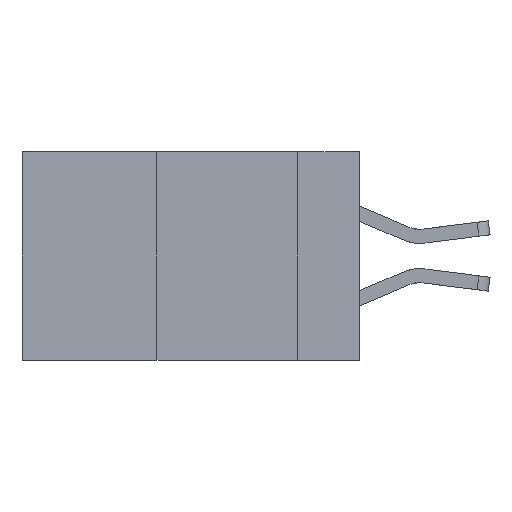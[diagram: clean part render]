
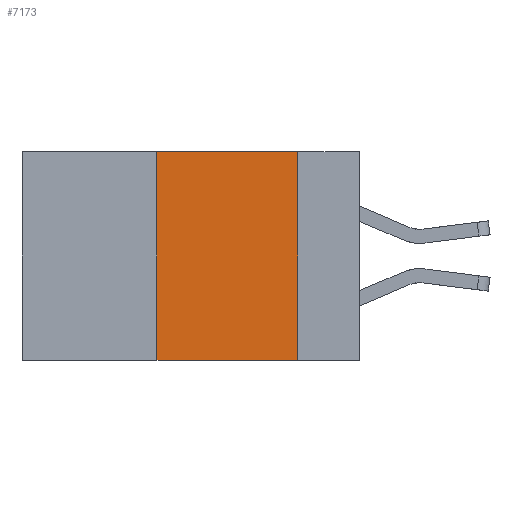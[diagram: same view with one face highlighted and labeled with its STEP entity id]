
A CAD part, left-side view. The second image highlights one B-rep face of the part: STEP entity #7173.
In plain terms, the highlighted planar face has unit normal (-1, 0, 0).
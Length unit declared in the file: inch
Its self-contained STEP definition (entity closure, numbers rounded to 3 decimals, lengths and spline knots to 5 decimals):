
#502 = DIRECTION ( 'NONE',  ( 0., -1., 0. ) ) ;
#1056 = DIRECTION ( 'NONE',  ( 0., -1., 0. ) ) ;
#1203 = CARTESIAN_POINT ( 'NONE',  ( 0., 0.11, 0. ) ) ;
#1405 = VECTOR ( 'NONE', #502, 39.37008 ) ;
#1530 = ORIENTED_EDGE ( 'NONE', *, *, #6728, .F. ) ;
#1878 = PLANE ( 'NONE',  #2097 ) ;
#2097 = AXIS2_PLACEMENT_3D ( 'NONE', #2658, #3518, #3548 ) ;
#2398 = ORIENTED_EDGE ( 'NONE', *, *, #4056, .T. ) ;
#2619 = ORIENTED_EDGE ( 'NONE', *, *, #3379, .F. ) ;
#2658 = CARTESIAN_POINT ( 'NONE',  ( 0., 0.6, 0. ) ) ;
#2898 = DIRECTION ( 'NONE',  ( 0., 0., 1. ) ) ;
#3379 = EDGE_CURVE ( 'NONE', #3621, #7911, #6817, .T. ) ;
#3418 = CARTESIAN_POINT ( 'NONE',  ( 0., 0.11, 0. ) ) ;
#3518 = DIRECTION ( 'NONE',  ( 1., 0., 0. ) ) ;
#3548 = DIRECTION ( 'NONE',  ( 0., 0., -1. ) ) ;
#3583 = CARTESIAN_POINT ( 'NONE',  ( 0., 0.6, 0. ) ) ;
#3621 = VERTEX_POINT ( 'NONE', #1203 ) ;
#3969 = DIRECTION ( 'NONE',  ( 0., 0., -1. ) ) ;
#4056 = EDGE_CURVE ( 'NONE', #10660, #7911, #10204, .T. ) ;
#4077 = CARTESIAN_POINT ( 'NONE',  ( 0., 0.36, -0.37 ) ) ;
#4946 = VERTEX_POINT ( 'NONE', #5895 ) ;
#5012 = CARTESIAN_POINT ( 'NONE',  ( 0., 0.6, -0.37 ) ) ;
#5367 = VECTOR ( 'NONE', #2898, 39.37008 ) ;
#5895 = CARTESIAN_POINT ( 'NONE',  ( 0., 0.36, 0. ) ) ;
#6003 = VECTOR ( 'NONE', #3969, 39.37008 ) ;
#6728 = EDGE_CURVE ( 'NONE', #10660, #4946, #8263, .T. ) ;
#6817 = LINE ( 'NONE', #3418, #6003 ) ;
#6995 = FACE_OUTER_BOUND ( 'NONE', #10558, .T. ) ;
#7173 = ADVANCED_FACE ( 'NONE', ( #6995 ), #1878, .F. ) ;
#7204 = CARTESIAN_POINT ( 'NONE',  ( 0., 0.36, 0. ) ) ;
#7911 = VERTEX_POINT ( 'NONE', #9703 ) ;
#8263 = LINE ( 'NONE', #7204, #5367 ) ;
#9167 = EDGE_CURVE ( 'NONE', #4946, #3621, #10472, .T. ) ;
#9289 = ORIENTED_EDGE ( 'NONE', *, *, #9167, .F. ) ;
#9405 = VECTOR ( 'NONE', #1056, 39.37008 ) ;
#9703 = CARTESIAN_POINT ( 'NONE',  ( 0., 0.11, -0.37 ) ) ;
#10204 = LINE ( 'NONE', #5012, #1405 ) ;
#10472 = LINE ( 'NONE', #3583, #9405 ) ;
#10558 = EDGE_LOOP ( 'NONE', ( #2619, #9289, #1530, #2398 ) ) ;
#10660 = VERTEX_POINT ( 'NONE', #4077 ) ;
